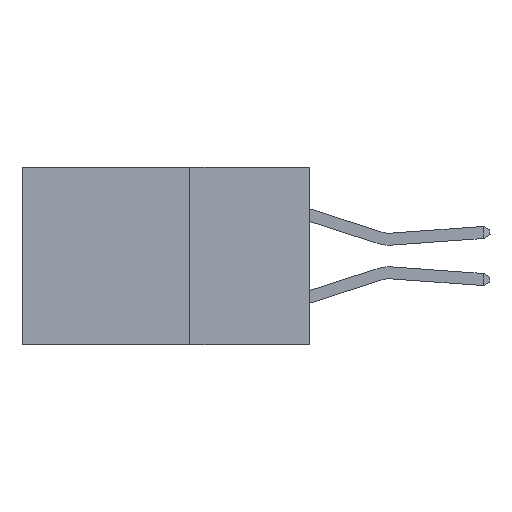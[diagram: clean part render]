
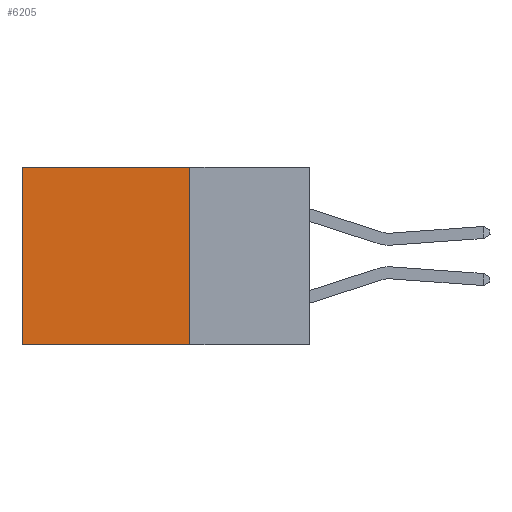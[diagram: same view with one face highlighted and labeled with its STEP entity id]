
A CAD part, left-side view. The second image highlights one B-rep face of the part: STEP entity #6205.
In plain terms, the highlighted planar face has unit normal (-1, 0, 0).
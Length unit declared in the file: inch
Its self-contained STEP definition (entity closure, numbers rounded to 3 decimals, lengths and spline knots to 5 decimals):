
#293 = CARTESIAN_POINT ( 'NONE',  ( 0.2615, 0.25, 0. ) ) ;
#350 = EDGE_LOOP ( 'NONE', ( #10362, #3977, #11761, #8280 ) ) ;
#383 = CARTESIAN_POINT ( 'NONE',  ( 0.2615, 0.6, -0.37 ) ) ;
#495 = DIRECTION ( 'NONE',  ( 0., 1., 0. ) ) ;
#567 = CARTESIAN_POINT ( 'NONE',  ( 0.2615, 0.25, -0.37 ) ) ;
#1694 = FACE_OUTER_BOUND ( 'NONE', #350, .T. ) ;
#2008 = VERTEX_POINT ( 'NONE', #8745 ) ;
#2144 = VERTEX_POINT ( 'NONE', #383 ) ;
#2352 = EDGE_CURVE ( 'NONE', #2008, #2144, #9460, .T. ) ;
#3306 = EDGE_CURVE ( 'NONE', #10010, #2144, #8416, .T. ) ;
#3977 = ORIENTED_EDGE ( 'NONE', *, *, #3306, .F. ) ;
#4095 = VECTOR ( 'NONE', #13571, 39.37008 ) ;
#4416 = VERTEX_POINT ( 'NONE', #293 ) ;
#5656 = LINE ( 'NONE', #12701, #11354 ) ;
#5893 = VECTOR ( 'NONE', #8236, 39.37008 ) ;
#6205 = ADVANCED_FACE ( 'NONE', ( #1694 ), #12730, .F. ) ;
#6677 = LINE ( 'NONE', #7276, #4095 ) ;
#7276 = CARTESIAN_POINT ( 'NONE',  ( 0.2615, 0.25, 0. ) ) ;
#8236 = DIRECTION ( 'NONE',  ( 0., 0., -1. ) ) ;
#8280 = ORIENTED_EDGE ( 'NONE', *, *, #13076, .T. ) ;
#8416 = LINE ( 'NONE', #567, #8751 ) ;
#8506 = CARTESIAN_POINT ( 'NONE',  ( 0.2615, 0.6, -0.37 ) ) ;
#8745 = CARTESIAN_POINT ( 'NONE',  ( 0.2615, 0.6, 0. ) ) ;
#8751 = VECTOR ( 'NONE', #495, 39.37008 ) ;
#9460 = LINE ( 'NONE', #8506, #5893 ) ;
#10010 = VERTEX_POINT ( 'NONE', #13676 ) ;
#10216 = AXIS2_PLACEMENT_3D ( 'NONE', #12610, #12592, #12554 ) ;
#10362 = ORIENTED_EDGE ( 'NONE', *, *, #2352, .T. ) ;
#11354 = VECTOR ( 'NONE', #13695, 39.37008 ) ;
#11761 = ORIENTED_EDGE ( 'NONE', *, *, #13151, .F. ) ;
#12554 = DIRECTION ( 'NONE',  ( 0., 0., -1. ) ) ;
#12592 = DIRECTION ( 'NONE',  ( 1., 0., 0. ) ) ;
#12610 = CARTESIAN_POINT ( 'NONE',  ( 0.2615, 0.25, -0.37 ) ) ;
#12701 = CARTESIAN_POINT ( 'NONE',  ( 0.2615, 0.25, -0.37 ) ) ;
#12730 = PLANE ( 'NONE',  #10216 ) ;
#13076 = EDGE_CURVE ( 'NONE', #4416, #2008, #6677, .T. ) ;
#13151 = EDGE_CURVE ( 'NONE', #4416, #10010, #5656, .T. ) ;
#13571 = DIRECTION ( 'NONE',  ( 0., 1., 0. ) ) ;
#13676 = CARTESIAN_POINT ( 'NONE',  ( 0.2615, 0.25, -0.37 ) ) ;
#13695 = DIRECTION ( 'NONE',  ( 0., 0., -1. ) ) ;
